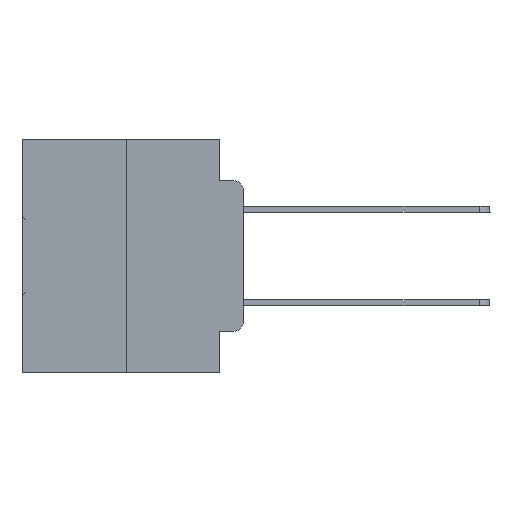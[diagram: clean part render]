
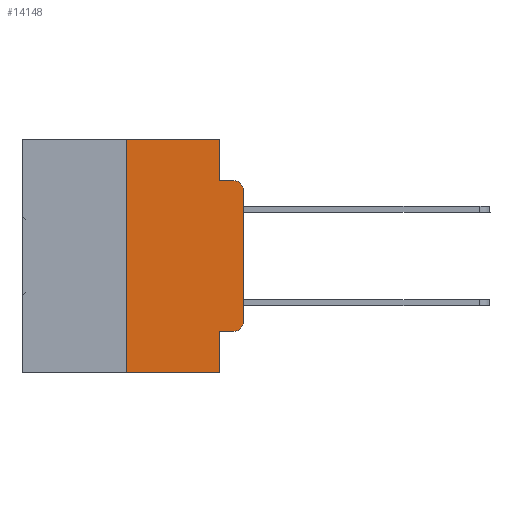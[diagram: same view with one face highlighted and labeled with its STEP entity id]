
A CAD part, left-side view. The second image highlights one B-rep face of the part: STEP entity #14148.
In plain terms, the highlighted planar face has unit normal (-1, 0, 0).
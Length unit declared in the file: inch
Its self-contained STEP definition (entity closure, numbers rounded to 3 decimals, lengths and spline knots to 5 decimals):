
#1273 = ORIENTED_EDGE ( 'NONE', *, *, #27975, .T. ) ;
#1303 = DIRECTION ( 'NONE',  ( 0., -1., 0. ) ) ;
#1697 = EDGE_CURVE ( 'NONE', #14445, #33093, #19001, .T. ) ;
#3047 = ORIENTED_EDGE ( 'NONE', *, *, #24256, .F. ) ;
#3360 = VECTOR ( 'NONE', #16472, 39.37008 ) ;
#3498 = VERTEX_POINT ( 'NONE', #20495 ) ;
#3575 = EDGE_CURVE ( 'NONE', #25351, #14445, #4377, .T. ) ;
#3716 = DIRECTION ( 'NONE',  ( 0., 0., -1. ) ) ;
#4250 = LINE ( 'NONE', #27517, #3360 ) ;
#4377 = LINE ( 'NONE', #34754, #32329 ) ;
#4396 = DIRECTION ( 'NONE',  ( -1., 0., 0. ) ) ;
#4821 = ORIENTED_EDGE ( 'NONE', *, *, #14910, .F. ) ;
#4981 = VECTOR ( 'NONE', #27349, 39.37008 ) ;
#5258 = VECTOR ( 'NONE', #34995, 39.37008 ) ;
#5264 = VECTOR ( 'NONE', #16670, 39.37008 ) ;
#6047 = CIRCLE ( 'NONE', #15336, 0.02 ) ;
#6144 = LINE ( 'NONE', #18432, #5258 ) ;
#6195 = CARTESIAN_POINT ( 'NONE',  ( 0., 0.473, -0.5 ) ) ;
#6592 = ORIENTED_EDGE ( 'NONE', *, *, #13019, .F. ) ;
#6909 = EDGE_CURVE ( 'NONE', #23017, #12407, #19948, .T. ) ;
#8366 = ORIENTED_EDGE ( 'NONE', *, *, #9258, .F. ) ;
#9258 = EDGE_CURVE ( 'NONE', #25351, #35605, #21504, .T. ) ;
#9265 = ORIENTED_EDGE ( 'NONE', *, *, #1697, .T. ) ;
#10057 = PLANE ( 'NONE',  #26262 ) ;
#11102 = CARTESIAN_POINT ( 'NONE',  ( 0., 0.25, 0. ) ) ;
#12293 = CARTESIAN_POINT ( 'NONE',  ( 0., 0., 0. ) ) ;
#12306 = ORIENTED_EDGE ( 'NONE', *, *, #6909, .F. ) ;
#12407 = VERTEX_POINT ( 'NONE', #22429 ) ;
#12891 = CARTESIAN_POINT ( 'NONE',  ( 0., 0.473, 0. ) ) ;
#13019 = EDGE_CURVE ( 'NONE', #13694, #23017, #13643, .T. ) ;
#13308 = CARTESIAN_POINT ( 'NONE',  ( 0., 0.473, 0. ) ) ;
#13424 = LINE ( 'NONE', #6195, #28258 ) ;
#13599 = DIRECTION ( 'NONE',  ( 0., 0., -1. ) ) ;
#13643 = LINE ( 'NONE', #11102, #5264 ) ;
#13694 = VERTEX_POINT ( 'NONE', #13777 ) ;
#13777 = CARTESIAN_POINT ( 'NONE',  ( 0., 0.25, -0.5 ) ) ;
#14148 = ADVANCED_FACE ( 'NONE', ( #22323 ), #10057, .F. ) ;
#14445 = VERTEX_POINT ( 'NONE', #28231 ) ;
#14910 = EDGE_CURVE ( 'NONE', #12407, #23395, #4250, .T. ) ;
#15336 = AXIS2_PLACEMENT_3D ( 'NONE', #21227, #4396, #24003 ) ;
#15733 = DIRECTION ( 'NONE',  ( 1., 0., 0. ) ) ;
#16472 = DIRECTION ( 'NONE',  ( 0., 0., -1. ) ) ;
#16670 = DIRECTION ( 'NONE',  ( 0., 0., 1. ) ) ;
#17079 = EDGE_LOOP ( 'NONE', ( #1273, #17175, #3047, #4821, #12306, #6592, #28883, #8366, #23261, #9265 ) ) ;
#17154 = CARTESIAN_POINT ( 'NONE',  ( 0., 0., -0.3915 ) ) ;
#17175 = ORIENTED_EDGE ( 'NONE', *, *, #26114, .T. ) ;
#17381 = LINE ( 'NONE', #12293, #23887 ) ;
#18432 = CARTESIAN_POINT ( 'NONE',  ( 0., 0.051, -0.0885 ) ) ;
#19001 = CIRCLE ( 'NONE', #32247, 0.02 ) ;
#19948 = LINE ( 'NONE', #13308, #4981 ) ;
#20495 = CARTESIAN_POINT ( 'NONE',  ( 0., 0., -0.1085 ) ) ;
#21227 = CARTESIAN_POINT ( 'NONE',  ( 0., 0.02, -0.1085 ) ) ;
#21504 = LINE ( 'NONE', #22040, #35347 ) ;
#21672 = CARTESIAN_POINT ( 'NONE',  ( 0., 0.02, -0.0885 ) ) ;
#22040 = CARTESIAN_POINT ( 'NONE',  ( 0., 0.051, 0. ) ) ;
#22323 = FACE_OUTER_BOUND ( 'NONE', #17079, .T. ) ;
#22338 = VERTEX_POINT ( 'NONE', #21672 ) ;
#22429 = CARTESIAN_POINT ( 'NONE',  ( 0., 0.051, 0. ) ) ;
#23001 = DIRECTION ( 'NONE',  ( 0., -1., 0. ) ) ;
#23017 = VERTEX_POINT ( 'NONE', #24539 ) ;
#23261 = ORIENTED_EDGE ( 'NONE', *, *, #3575, .T. ) ;
#23395 = VERTEX_POINT ( 'NONE', #35014 ) ;
#23887 = VECTOR ( 'NONE', #26218, 39.37008 ) ;
#24003 = DIRECTION ( 'NONE',  ( 0., 0., -1. ) ) ;
#24256 = EDGE_CURVE ( 'NONE', #23395, #22338, #6144, .T. ) ;
#24539 = CARTESIAN_POINT ( 'NONE',  ( 0., 0.25, 0. ) ) ;
#25351 = VERTEX_POINT ( 'NONE', #31673 ) ;
#26114 = EDGE_CURVE ( 'NONE', #3498, #22338, #6047, .T. ) ;
#26218 = DIRECTION ( 'NONE',  ( 0., 0., 1. ) ) ;
#26262 = AXIS2_PLACEMENT_3D ( 'NONE', #12891, #15733, #35119 ) ;
#27349 = DIRECTION ( 'NONE',  ( 0., -1., 0. ) ) ;
#27517 = CARTESIAN_POINT ( 'NONE',  ( 0., 0.051, 0. ) ) ;
#27519 = CARTESIAN_POINT ( 'NONE',  ( 0., 0.051, -0.5 ) ) ;
#27975 = EDGE_CURVE ( 'NONE', #33093, #3498, #17381, .T. ) ;
#28231 = CARTESIAN_POINT ( 'NONE',  ( 0., 0.02, -0.4115 ) ) ;
#28258 = VECTOR ( 'NONE', #23001, 39.37008 ) ;
#28883 = ORIENTED_EDGE ( 'NONE', *, *, #35853, .T. ) ;
#29418 = DIRECTION ( 'NONE',  ( -1., 0., 0. ) ) ;
#29495 = CARTESIAN_POINT ( 'NONE',  ( 0., 0.02, -0.3915 ) ) ;
#31673 = CARTESIAN_POINT ( 'NONE',  ( 0., 0.051, -0.4115 ) ) ;
#32247 = AXIS2_PLACEMENT_3D ( 'NONE', #29495, #29418, #3716 ) ;
#32329 = VECTOR ( 'NONE', #1303, 39.37008 ) ;
#33093 = VERTEX_POINT ( 'NONE', #17154 ) ;
#34754 = CARTESIAN_POINT ( 'NONE',  ( 0., 0.051, -0.4115 ) ) ;
#34995 = DIRECTION ( 'NONE',  ( 0., -1., 0. ) ) ;
#35014 = CARTESIAN_POINT ( 'NONE',  ( 0., 0.051, -0.0885 ) ) ;
#35119 = DIRECTION ( 'NONE',  ( 0., 0., -1. ) ) ;
#35347 = VECTOR ( 'NONE', #13599, 39.37008 ) ;
#35605 = VERTEX_POINT ( 'NONE', #27519 ) ;
#35853 = EDGE_CURVE ( 'NONE', #13694, #35605, #13424, .T. ) ;
